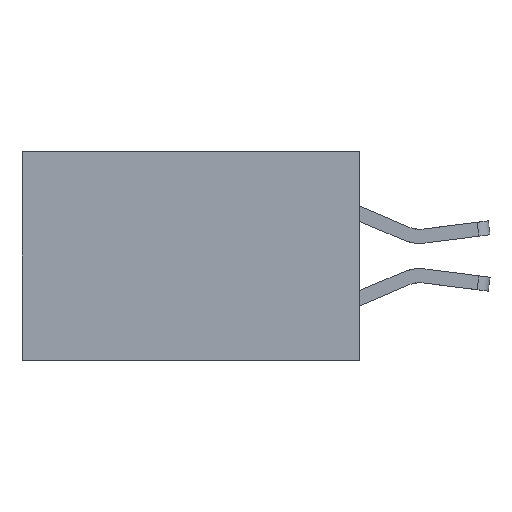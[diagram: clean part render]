
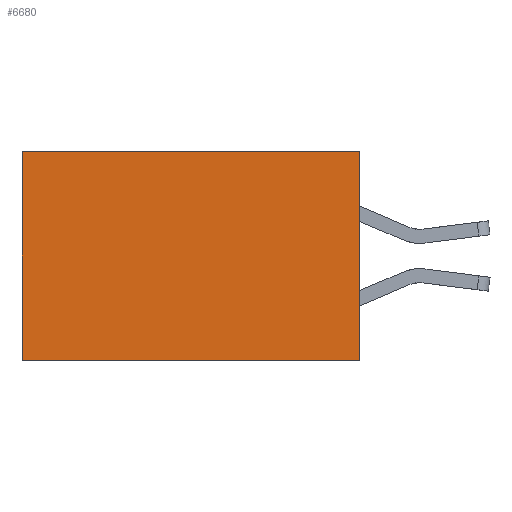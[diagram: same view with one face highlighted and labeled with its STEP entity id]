
A CAD part, left-side view. The second image highlights one B-rep face of the part: STEP entity #6680.
In plain terms, the highlighted planar face has unit normal (-1, 0, 0).
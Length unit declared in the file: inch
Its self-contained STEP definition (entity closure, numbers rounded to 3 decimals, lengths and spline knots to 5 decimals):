
#27 = EDGE_CURVE ( 'NONE', #438, #8773, #5085, .T. ) ;
#92 = DIRECTION ( 'NONE',  ( 0., 0., -1. ) ) ;
#438 = VERTEX_POINT ( 'NONE', #1570 ) ;
#752 = CARTESIAN_POINT ( 'NONE',  ( 0.2875, 0., -0.37 ) ) ;
#878 = VECTOR ( 'NONE', #6503, 39.37008 ) ;
#1031 = VERTEX_POINT ( 'NONE', #2198 ) ;
#1570 = CARTESIAN_POINT ( 'NONE',  ( 0.2875, 0., -0.37 ) ) ;
#2198 = CARTESIAN_POINT ( 'NONE',  ( 0.2875, 0.6, 0. ) ) ;
#2510 = ORIENTED_EDGE ( 'NONE', *, *, #6281, .T. ) ;
#2556 = AXIS2_PLACEMENT_3D ( 'NONE', #8301, #6981, #92 ) ;
#2693 = EDGE_CURVE ( 'NONE', #5036, #438, #6948, .T. ) ;
#2800 = DIRECTION ( 'NONE',  ( 0., 0., -1. ) ) ;
#2905 = ORIENTED_EDGE ( 'NONE', *, *, #6825, .T. ) ;
#3136 = EDGE_LOOP ( 'NONE', ( #2510, #8510, #3788, #2905 ) ) ;
#3577 = PLANE ( 'NONE',  #2556 ) ;
#3649 = CARTESIAN_POINT ( 'NONE',  ( 0.2875, 0., 0. ) ) ;
#3788 = ORIENTED_EDGE ( 'NONE', *, *, #2693, .F. ) ;
#4432 = CARTESIAN_POINT ( 'NONE',  ( 0.2875, 0., 0. ) ) ;
#4804 = CARTESIAN_POINT ( 'NONE',  ( 0.2875, 0.6, -0.37 ) ) ;
#4832 = CARTESIAN_POINT ( 'NONE',  ( 0.2875, 0.6, 0. ) ) ;
#5036 = VERTEX_POINT ( 'NONE', #6334 ) ;
#5085 = LINE ( 'NONE', #752, #5304 ) ;
#5304 = VECTOR ( 'NONE', #7671, 39.37008 ) ;
#6281 = EDGE_CURVE ( 'NONE', #1031, #8773, #6765, .T. ) ;
#6334 = CARTESIAN_POINT ( 'NONE',  ( 0.2875, 0., 0. ) ) ;
#6503 = DIRECTION ( 'NONE',  ( 0., 1., 0. ) ) ;
#6523 = VECTOR ( 'NONE', #8425, 39.37008 ) ;
#6680 = ADVANCED_FACE ( 'NONE', ( #8022 ), #3577, .F. ) ;
#6765 = LINE ( 'NONE', #4832, #8337 ) ;
#6825 = EDGE_CURVE ( 'NONE', #5036, #1031, #8666, .T. ) ;
#6948 = LINE ( 'NONE', #3649, #6523 ) ;
#6981 = DIRECTION ( 'NONE',  ( 1., 0., 0. ) ) ;
#7671 = DIRECTION ( 'NONE',  ( 0., 1., 0. ) ) ;
#8022 = FACE_OUTER_BOUND ( 'NONE', #3136, .T. ) ;
#8301 = CARTESIAN_POINT ( 'NONE',  ( 0.2875, 0., 0. ) ) ;
#8337 = VECTOR ( 'NONE', #2800, 39.37008 ) ;
#8425 = DIRECTION ( 'NONE',  ( 0., 0., -1. ) ) ;
#8510 = ORIENTED_EDGE ( 'NONE', *, *, #27, .F. ) ;
#8666 = LINE ( 'NONE', #4432, #878 ) ;
#8773 = VERTEX_POINT ( 'NONE', #4804 ) ;
